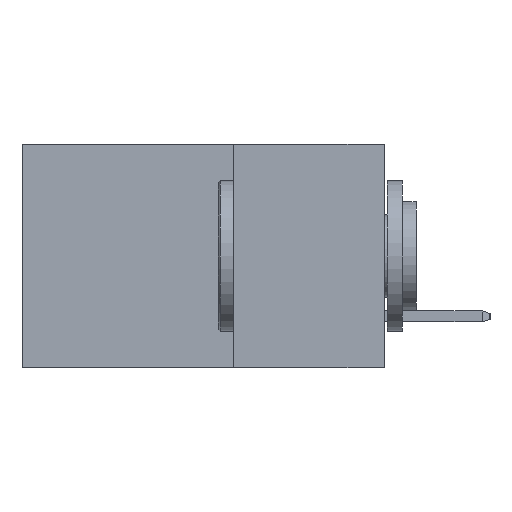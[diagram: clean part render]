
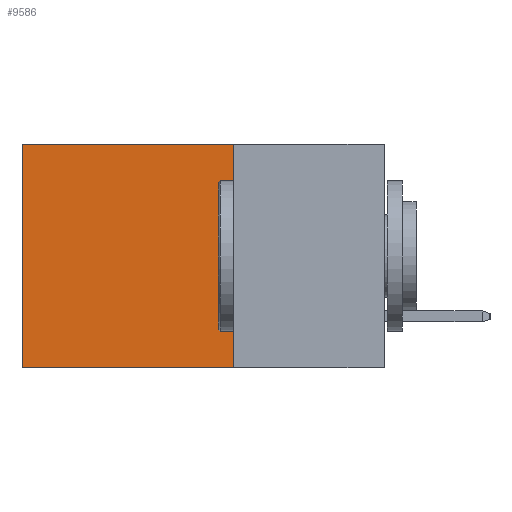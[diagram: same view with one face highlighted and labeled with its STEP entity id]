
A CAD part, left-side view. The second image highlights one B-rep face of the part: STEP entity #9586.
In plain terms, the highlighted planar face has unit normal (-1, 0, 0).
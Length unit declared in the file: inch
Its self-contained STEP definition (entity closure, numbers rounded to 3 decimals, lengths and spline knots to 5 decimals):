
#152 = VERTEX_POINT ( 'NONE', #13079 ) ;
#1051 = CARTESIAN_POINT ( 'NONE',  ( 0.2615, 0.25, -0.37 ) ) ;
#1112 = VERTEX_POINT ( 'NONE', #8387 ) ;
#1457 = EDGE_CURVE ( 'NONE', #3925, #1670, #12082, .T. ) ;
#1670 = VERTEX_POINT ( 'NONE', #7828 ) ;
#2355 = DIRECTION ( 'NONE',  ( 1., 0., 0. ) ) ;
#2481 = EDGE_CURVE ( 'NONE', #1670, #152, #6411, .T. ) ;
#2587 = CARTESIAN_POINT ( 'NONE',  ( 0.2615, 0.25, -0.37 ) ) ;
#2959 = CARTESIAN_POINT ( 'NONE',  ( 0.2615, 0.25, 0. ) ) ;
#3925 = VERTEX_POINT ( 'NONE', #5000 ) ;
#4121 = ORIENTED_EDGE ( 'NONE', *, *, #14521, .T. ) ;
#4171 = DIRECTION ( 'NONE',  ( 0., 1., 0. ) ) ;
#4192 = ORIENTED_EDGE ( 'NONE', *, *, #2481, .F. ) ;
#4796 = CARTESIAN_POINT ( 'NONE',  ( 0.2615, 0.25, -0.37 ) ) ;
#5000 = CARTESIAN_POINT ( 'NONE',  ( 0.2615, 0.25, 0. ) ) ;
#5182 = EDGE_LOOP ( 'NONE', ( #4121, #4192, #10257, #15167 ) ) ;
#5438 = DIRECTION ( 'NONE',  ( 0., 0., -1. ) ) ;
#6408 = LINE ( 'NONE', #12451, #14766 ) ;
#6411 = LINE ( 'NONE', #2587, #15116 ) ;
#6715 = VECTOR ( 'NONE', #4171, 39.37008 ) ;
#7099 = LINE ( 'NONE', #2959, #6715 ) ;
#7828 = CARTESIAN_POINT ( 'NONE',  ( 0.2615, 0.25, -0.37 ) ) ;
#8087 = EDGE_CURVE ( 'NONE', #3925, #1112, #7099, .T. ) ;
#8387 = CARTESIAN_POINT ( 'NONE',  ( 0.2615, 0.6, 0. ) ) ;
#9561 = DIRECTION ( 'NONE',  ( 0., 0., -1. ) ) ;
#9586 = ADVANCED_FACE ( 'NONE', ( #10377 ), #9612, .F. ) ;
#9612 = PLANE ( 'NONE',  #12635 ) ;
#10257 = ORIENTED_EDGE ( 'NONE', *, *, #1457, .F. ) ;
#10377 = FACE_OUTER_BOUND ( 'NONE', #5182, .T. ) ;
#10794 = DIRECTION ( 'NONE',  ( 0., 0., -1. ) ) ;
#11663 = DIRECTION ( 'NONE',  ( 0., 1., 0. ) ) ;
#12082 = LINE ( 'NONE', #4796, #14642 ) ;
#12451 = CARTESIAN_POINT ( 'NONE',  ( 0.2615, 0.6, -0.37 ) ) ;
#12635 = AXIS2_PLACEMENT_3D ( 'NONE', #1051, #2355, #10794 ) ;
#13079 = CARTESIAN_POINT ( 'NONE',  ( 0.2615, 0.6, -0.37 ) ) ;
#14521 = EDGE_CURVE ( 'NONE', #1112, #152, #6408, .T. ) ;
#14642 = VECTOR ( 'NONE', #9561, 39.37008 ) ;
#14766 = VECTOR ( 'NONE', #5438, 39.37008 ) ;
#15116 = VECTOR ( 'NONE', #11663, 39.37008 ) ;
#15167 = ORIENTED_EDGE ( 'NONE', *, *, #8087, .T. ) ;
